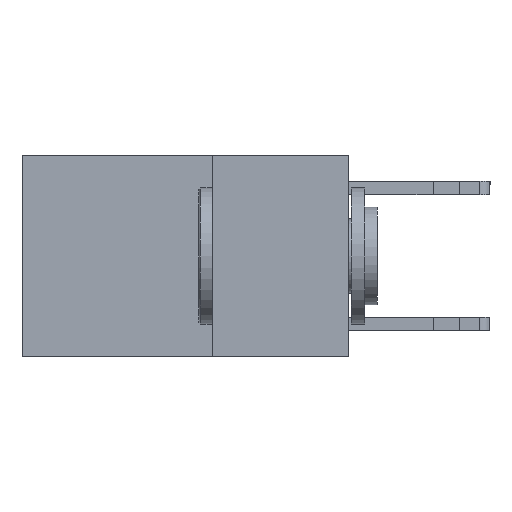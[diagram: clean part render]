
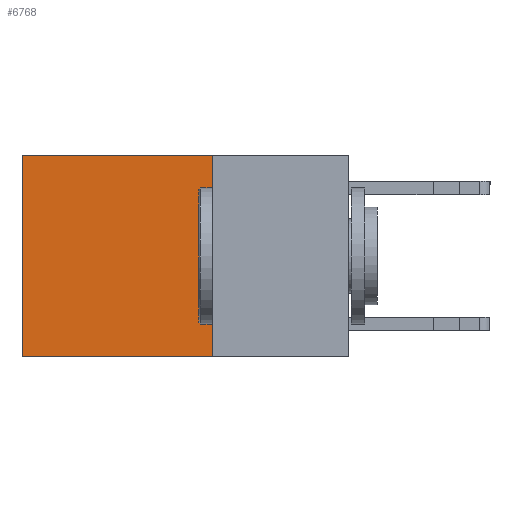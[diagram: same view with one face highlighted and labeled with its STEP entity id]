
A CAD part, left-side view. The second image highlights one B-rep face of the part: STEP entity #6768.
In plain terms, the highlighted planar face has unit normal (-1, 0, 0).
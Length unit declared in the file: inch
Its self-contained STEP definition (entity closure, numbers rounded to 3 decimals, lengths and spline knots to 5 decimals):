
#236 = DIRECTION ( 'NONE',  ( 0., 0., -1. ) ) ;
#684 = EDGE_CURVE ( 'NONE', #2831, #10160, #898, .T. ) ;
#761 = EDGE_CURVE ( 'NONE', #11611, #2831, #7460, .T. ) ;
#898 = LINE ( 'NONE', #8347, #9977 ) ;
#917 = CARTESIAN_POINT ( 'NONE',  ( 0.2625, 0.25, 0. ) ) ;
#1165 = VECTOR ( 'NONE', #10397, 39.37008 ) ;
#1231 = VECTOR ( 'NONE', #7271, 39.37008 ) ;
#1604 = DIRECTION ( 'NONE',  ( 0., 1., 0. ) ) ;
#2444 = ORIENTED_EDGE ( 'NONE', *, *, #11259, .T. ) ;
#2831 = VERTEX_POINT ( 'NONE', #6884 ) ;
#3417 = CARTESIAN_POINT ( 'NONE',  ( 0.2625, 0.25, 0. ) ) ;
#4165 = LINE ( 'NONE', #3417, #1231 ) ;
#4207 = CARTESIAN_POINT ( 'NONE',  ( 0.2625, 0.6, -0.37 ) ) ;
#5093 = VECTOR ( 'NONE', #7518, 39.37008 ) ;
#5529 = CARTESIAN_POINT ( 'NONE',  ( 0.2625, 0.25, 0. ) ) ;
#5776 = ORIENTED_EDGE ( 'NONE', *, *, #12265, .T. ) ;
#6524 = CARTESIAN_POINT ( 'NONE',  ( 0.2625, 0.6, 0. ) ) ;
#6597 = DIRECTION ( 'NONE',  ( 1., 0., 0. ) ) ;
#6768 = ADVANCED_FACE ( 'NONE', ( #8883 ), #11538, .F. ) ;
#6884 = CARTESIAN_POINT ( 'NONE',  ( 0.2625, 0.25, -0.37 ) ) ;
#6975 = EDGE_LOOP ( 'NONE', ( #5776, #11473, #11555, #2444 ) ) ;
#7120 = CARTESIAN_POINT ( 'NONE',  ( 0.2625, 0.6, 0. ) ) ;
#7271 = DIRECTION ( 'NONE',  ( 0., 1., 0. ) ) ;
#7460 = LINE ( 'NONE', #5529, #5093 ) ;
#7518 = DIRECTION ( 'NONE',  ( 0., 0., -1. ) ) ;
#8347 = CARTESIAN_POINT ( 'NONE',  ( 0.2625, 0.25, -0.37 ) ) ;
#8883 = FACE_OUTER_BOUND ( 'NONE', #6975, .T. ) ;
#8992 = VERTEX_POINT ( 'NONE', #7120 ) ;
#9233 = AXIS2_PLACEMENT_3D ( 'NONE', #917, #6597, #236 ) ;
#9977 = VECTOR ( 'NONE', #1604, 39.37008 ) ;
#10160 = VERTEX_POINT ( 'NONE', #4207 ) ;
#10397 = DIRECTION ( 'NONE',  ( 0., 0., -1. ) ) ;
#10992 = CARTESIAN_POINT ( 'NONE',  ( 0.2625, 0.25, 0. ) ) ;
#11259 = EDGE_CURVE ( 'NONE', #11611, #8992, #4165, .T. ) ;
#11349 = LINE ( 'NONE', #6524, #1165 ) ;
#11473 = ORIENTED_EDGE ( 'NONE', *, *, #684, .F. ) ;
#11538 = PLANE ( 'NONE',  #9233 ) ;
#11555 = ORIENTED_EDGE ( 'NONE', *, *, #761, .F. ) ;
#11611 = VERTEX_POINT ( 'NONE', #10992 ) ;
#12265 = EDGE_CURVE ( 'NONE', #8992, #10160, #11349, .T. ) ;
